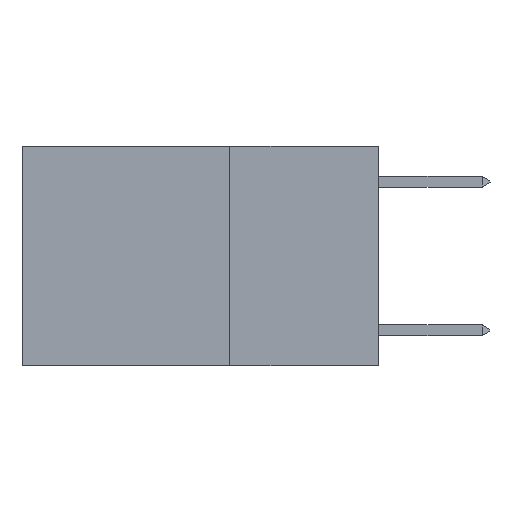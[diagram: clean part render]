
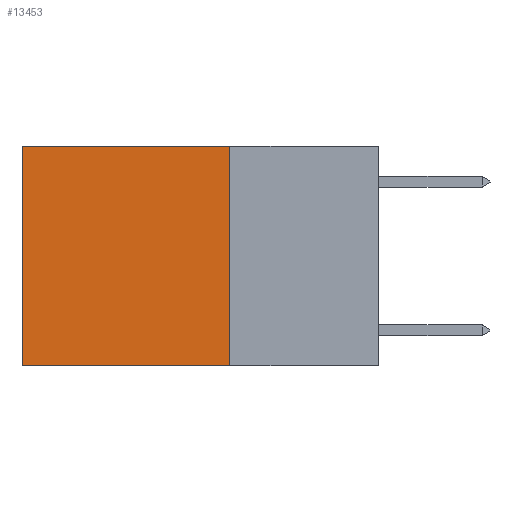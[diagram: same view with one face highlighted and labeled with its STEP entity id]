
A CAD part, left-side view. The second image highlights one B-rep face of the part: STEP entity #13453.
In plain terms, the highlighted planar face has unit normal (-1, 0, 0).
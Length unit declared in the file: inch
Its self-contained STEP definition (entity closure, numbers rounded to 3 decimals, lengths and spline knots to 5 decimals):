
#43 = VERTEX_POINT ( 'NONE', #13877 ) ;
#574 = LINE ( 'NONE', #3274, #6351 ) ;
#787 = CARTESIAN_POINT ( 'NONE',  ( 0.2625, 0.6, -0.37 ) ) ;
#1048 = FACE_OUTER_BOUND ( 'NONE', #1556, .T. ) ;
#1267 = EDGE_CURVE ( 'NONE', #6497, #8412, #10439, .T. ) ;
#1556 = EDGE_LOOP ( 'NONE', ( #5962, #4015, #12893, #11323 ) ) ;
#1750 = CARTESIAN_POINT ( 'NONE',  ( 0.2625, 0.25, 0. ) ) ;
#1972 = CARTESIAN_POINT ( 'NONE',  ( 0.2625, 0.6, 0. ) ) ;
#3274 = CARTESIAN_POINT ( 'NONE',  ( 0.2625, 0.25, 0. ) ) ;
#3319 = VECTOR ( 'NONE', #6824, 39.37008 ) ;
#4015 = ORIENTED_EDGE ( 'NONE', *, *, #8595, .F. ) ;
#5141 = CARTESIAN_POINT ( 'NONE',  ( 0.2625, 0.25, -0.37 ) ) ;
#5697 = CARTESIAN_POINT ( 'NONE',  ( 0.2625, 0.6, 0. ) ) ;
#5962 = ORIENTED_EDGE ( 'NONE', *, *, #1267, .T. ) ;
#6083 = DIRECTION ( 'NONE',  ( 0., 0., -1. ) ) ;
#6351 = VECTOR ( 'NONE', #9997, 39.37008 ) ;
#6497 = VERTEX_POINT ( 'NONE', #1972 ) ;
#6824 = DIRECTION ( 'NONE',  ( 0., 1., 0. ) ) ;
#7813 = EDGE_CURVE ( 'NONE', #43, #6497, #574, .T. ) ;
#8260 = VERTEX_POINT ( 'NONE', #5141 ) ;
#8412 = VERTEX_POINT ( 'NONE', #787 ) ;
#8595 = EDGE_CURVE ( 'NONE', #8260, #8412, #14484, .T. ) ;
#9839 = DIRECTION ( 'NONE',  ( 0., 0., -1. ) ) ;
#9997 = DIRECTION ( 'NONE',  ( 0., 1., 0. ) ) ;
#10118 = DIRECTION ( 'NONE',  ( 0., 0., -1. ) ) ;
#10439 = LINE ( 'NONE', #5697, #13386 ) ;
#10492 = PLANE ( 'NONE',  #13602 ) ;
#11323 = ORIENTED_EDGE ( 'NONE', *, *, #7813, .T. ) ;
#11463 = VECTOR ( 'NONE', #10118, 39.37008 ) ;
#11587 = CARTESIAN_POINT ( 'NONE',  ( 0.2625, 0.25, 0. ) ) ;
#11906 = EDGE_CURVE ( 'NONE', #43, #8260, #14414, .T. ) ;
#12702 = DIRECTION ( 'NONE',  ( 1., 0., 0. ) ) ;
#12893 = ORIENTED_EDGE ( 'NONE', *, *, #11906, .F. ) ;
#13386 = VECTOR ( 'NONE', #9839, 39.37008 ) ;
#13453 = ADVANCED_FACE ( 'NONE', ( #1048 ), #10492, .F. ) ;
#13476 = CARTESIAN_POINT ( 'NONE',  ( 0.2625, 0.25, -0.37 ) ) ;
#13602 = AXIS2_PLACEMENT_3D ( 'NONE', #11587, #12702, #6083 ) ;
#13877 = CARTESIAN_POINT ( 'NONE',  ( 0.2625, 0.25, 0. ) ) ;
#14414 = LINE ( 'NONE', #1750, #11463 ) ;
#14484 = LINE ( 'NONE', #13476, #3319 ) ;
